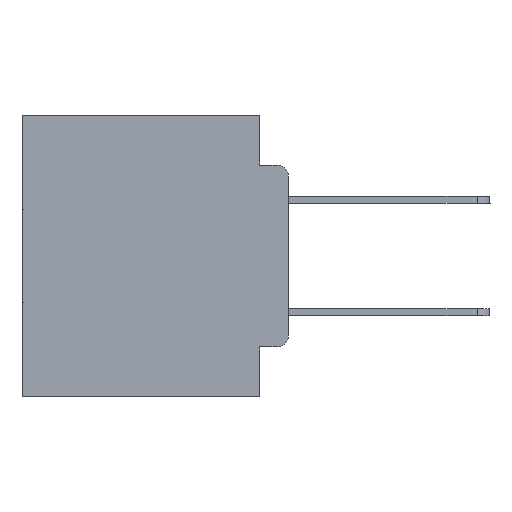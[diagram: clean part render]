
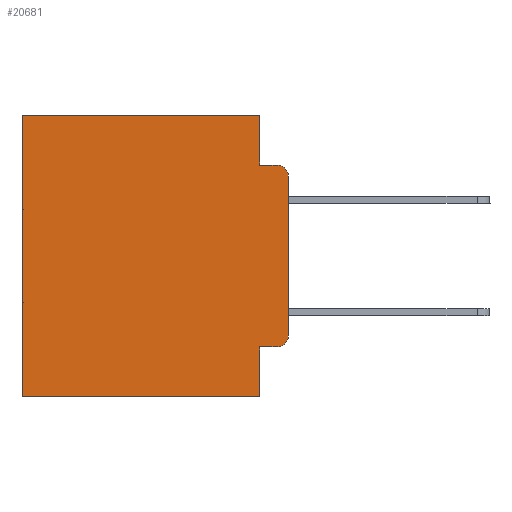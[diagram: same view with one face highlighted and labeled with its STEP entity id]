
A CAD part, left-side view. The second image highlights one B-rep face of the part: STEP entity #20681.
In plain terms, the highlighted planar face has unit normal (-1, 0, 0).
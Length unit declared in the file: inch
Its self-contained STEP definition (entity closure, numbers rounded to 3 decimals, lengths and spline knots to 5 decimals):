
#116 = EDGE_CURVE ( 'NONE', #1258, #27983, #13129, .T. ) ;
#715 = EDGE_CURVE ( 'NONE', #5239, #7110, #29740, .T. ) ;
#904 = CARTESIAN_POINT ( 'NONE',  ( 0.298, 0., 0. ) ) ;
#1056 = LINE ( 'NONE', #904, #18248 ) ;
#1241 = CARTESIAN_POINT ( 'NONE',  ( 0.298, 0.051, -0.0885 ) ) ;
#1258 = VERTEX_POINT ( 'NONE', #13948 ) ;
#1545 = DIRECTION ( 'NONE',  ( 0., -1., 0. ) ) ;
#1816 = DIRECTION ( 'NONE',  ( 0., -1., 0. ) ) ;
#1831 = EDGE_CURVE ( 'NONE', #5239, #16548, #13095, .T. ) ;
#1927 = ORIENTED_EDGE ( 'NONE', *, *, #20379, .T. ) ;
#2104 = CARTESIAN_POINT ( 'NONE',  ( 0.298, 0.051, -0.4115 ) ) ;
#2351 = CIRCLE ( 'NONE', #10148, 0.02 ) ;
#2623 = DIRECTION ( 'NONE',  ( 0., 1., 0. ) ) ;
#2647 = ORIENTED_EDGE ( 'NONE', *, *, #715, .T. ) ;
#3125 = VECTOR ( 'NONE', #10651, 39.37008 ) ;
#3436 = CARTESIAN_POINT ( 'NONE',  ( 0.298, 0.02, -0.4115 ) ) ;
#3529 = VECTOR ( 'NONE', #18348, 39.37008 ) ;
#3895 = LINE ( 'NONE', #22773, #3529 ) ;
#4893 = CARTESIAN_POINT ( 'NONE',  ( 0.298, 0.02, -0.3915 ) ) ;
#5239 = VERTEX_POINT ( 'NONE', #5458 ) ;
#5458 = CARTESIAN_POINT ( 'NONE',  ( 0.298, 0.051, -0.4115 ) ) ;
#5953 = CARTESIAN_POINT ( 'NONE',  ( 0.298, 0.051, 0. ) ) ;
#6248 = CARTESIAN_POINT ( 'NONE',  ( 0.298, 0.051, 0. ) ) ;
#6539 = CARTESIAN_POINT ( 'NONE',  ( 0.298, 0.051, -0.5 ) ) ;
#6566 = DIRECTION ( 'NONE',  ( -1., 0., 0. ) ) ;
#6953 = AXIS2_PLACEMENT_3D ( 'NONE', #10239, #6566, #17852 ) ;
#6976 = VECTOR ( 'NONE', #1816, 39.37008 ) ;
#7110 = VERTEX_POINT ( 'NONE', #3436 ) ;
#7352 = VERTEX_POINT ( 'NONE', #15921 ) ;
#7629 = DIRECTION ( 'NONE',  ( -1., 0., 0. ) ) ;
#8545 = CARTESIAN_POINT ( 'NONE',  ( 0.298, 0., 0. ) ) ;
#8978 = ORIENTED_EDGE ( 'NONE', *, *, #12171, .T. ) ;
#9037 = CARTESIAN_POINT ( 'NONE',  ( 0.298, 0.473, -0.5 ) ) ;
#9331 = LINE ( 'NONE', #23498, #17228 ) ;
#10148 = AXIS2_PLACEMENT_3D ( 'NONE', #4893, #7629, #16904 ) ;
#10239 = CARTESIAN_POINT ( 'NONE',  ( 0.298, 0.02, -0.1085 ) ) ;
#10325 = ORIENTED_EDGE ( 'NONE', *, *, #14301, .F. ) ;
#10651 = DIRECTION ( 'NONE',  ( 0., 0., -1. ) ) ;
#12171 = EDGE_CURVE ( 'NONE', #7352, #24244, #3895, .T. ) ;
#12835 = EDGE_CURVE ( 'NONE', #18751, #27983, #25926, .T. ) ;
#12980 = CARTESIAN_POINT ( 'NONE',  ( 0.298, 0., -0.1085 ) ) ;
#13095 = LINE ( 'NONE', #5953, #3125 ) ;
#13129 = LINE ( 'NONE', #1241, #14053 ) ;
#13408 = DIRECTION ( 'NONE',  ( 1., 0., 0. ) ) ;
#13513 = ORIENTED_EDGE ( 'NONE', *, *, #16442, .T. ) ;
#13585 = AXIS2_PLACEMENT_3D ( 'NONE', #8545, #13408, #17828 ) ;
#13946 = EDGE_CURVE ( 'NONE', #16548, #24244, #9331, .T. ) ;
#13948 = CARTESIAN_POINT ( 'NONE',  ( 0.298, 0.051, -0.0885 ) ) ;
#14053 = VECTOR ( 'NONE', #1545, 39.37008 ) ;
#14301 = EDGE_CURVE ( 'NONE', #20708, #1258, #25009, .T. ) ;
#15873 = CARTESIAN_POINT ( 'NONE',  ( 0.298, 0.051, 0. ) ) ;
#15921 = CARTESIAN_POINT ( 'NONE',  ( 0.298, 0.473, 0. ) ) ;
#16442 = EDGE_CURVE ( 'NONE', #20708, #7352, #1056, .T. ) ;
#16548 = VERTEX_POINT ( 'NONE', #6539 ) ;
#16904 = DIRECTION ( 'NONE',  ( 0., 0., -1. ) ) ;
#17228 = VECTOR ( 'NONE', #2623, 39.37008 ) ;
#17258 = VECTOR ( 'NONE', #22854, 39.37008 ) ;
#17511 = DIRECTION ( 'NONE',  ( 0., 1., 0. ) ) ;
#17828 = DIRECTION ( 'NONE',  ( 0., 0., -1. ) ) ;
#17852 = DIRECTION ( 'NONE',  ( 0., 0., -1. ) ) ;
#18248 = VECTOR ( 'NONE', #17511, 39.37008 ) ;
#18348 = DIRECTION ( 'NONE',  ( 0., 0., -1. ) ) ;
#18351 = CARTESIAN_POINT ( 'NONE',  ( 0.298, 0., 0. ) ) ;
#18751 = VERTEX_POINT ( 'NONE', #12980 ) ;
#18872 = VERTEX_POINT ( 'NONE', #27483 ) ;
#19622 = ORIENTED_EDGE ( 'NONE', *, *, #29783, .F. ) ;
#19648 = ORIENTED_EDGE ( 'NONE', *, *, #13946, .F. ) ;
#19772 = EDGE_LOOP ( 'NONE', ( #19622, #21959, #20501, #10325, #13513, #8978, #19648, #21896, #2647, #1927 ) ) ;
#20121 = FACE_OUTER_BOUND ( 'NONE', #19772, .T. ) ;
#20379 = EDGE_CURVE ( 'NONE', #7110, #18872, #2351, .T. ) ;
#20501 = ORIENTED_EDGE ( 'NONE', *, *, #116, .F. ) ;
#20681 = ADVANCED_FACE ( 'NONE', ( #20121 ), #29455, .F. ) ;
#20708 = VERTEX_POINT ( 'NONE', #6248 ) ;
#21896 = ORIENTED_EDGE ( 'NONE', *, *, #1831, .F. ) ;
#21959 = ORIENTED_EDGE ( 'NONE', *, *, #12835, .T. ) ;
#22773 = CARTESIAN_POINT ( 'NONE',  ( 0.298, 0.473, 0. ) ) ;
#22854 = DIRECTION ( 'NONE',  ( 0., 0., -1. ) ) ;
#23498 = CARTESIAN_POINT ( 'NONE',  ( 0.298, 0., -0.5 ) ) ;
#24244 = VERTEX_POINT ( 'NONE', #9037 ) ;
#25009 = LINE ( 'NONE', #15873, #17258 ) ;
#25662 = DIRECTION ( 'NONE',  ( 0., 0., -1. ) ) ;
#25856 = CARTESIAN_POINT ( 'NONE',  ( 0.298, 0.02, -0.0885 ) ) ;
#25926 = CIRCLE ( 'NONE', #6953, 0.02 ) ;
#27483 = CARTESIAN_POINT ( 'NONE',  ( 0.298, 0., -0.3915 ) ) ;
#27540 = LINE ( 'NONE', #18351, #29895 ) ;
#27983 = VERTEX_POINT ( 'NONE', #25856 ) ;
#29455 = PLANE ( 'NONE',  #13585 ) ;
#29740 = LINE ( 'NONE', #2104, #6976 ) ;
#29783 = EDGE_CURVE ( 'NONE', #18751, #18872, #27540, .T. ) ;
#29895 = VECTOR ( 'NONE', #25662, 39.37008 ) ;
